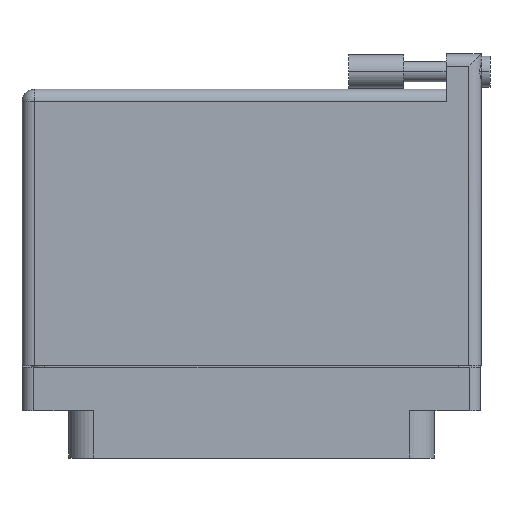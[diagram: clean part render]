
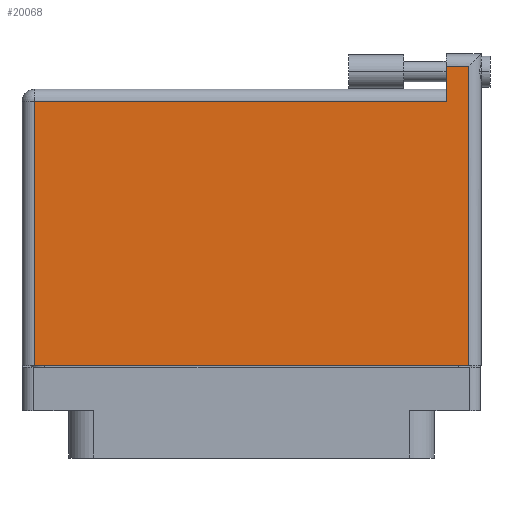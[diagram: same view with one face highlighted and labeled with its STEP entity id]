
A CAD part, front view. The second image highlights one B-rep face of the part: STEP entity #20068.
In plain terms, the highlighted face is planar.
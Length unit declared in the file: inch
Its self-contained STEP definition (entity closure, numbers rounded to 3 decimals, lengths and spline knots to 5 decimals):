
#1791 = LINE ( 'NONE', #7025, #42059 ) ;
#1835 = EDGE_CURVE ( 'NONE', #20853, #13419, #1791, .T. ) ;
#2866 = CARTESIAN_POINT ( 'NONE',  ( -1.23, -0.1, 0.4495 ) ) ;
#3007 = DIRECTION ( 'NONE',  ( -1., 0., 0. ) ) ;
#3185 = CARTESIAN_POINT ( 'NONE',  ( 1.103, 1.666, 0.4495 ) ) ;
#3357 = CARTESIAN_POINT ( 'NONE',  ( -1.3, 1.396, 0.4495 ) ) ;
#3384 = CARTESIAN_POINT ( 'NONE',  ( -1.23, -0.1, 0.4495 ) ) ;
#4077 = LINE ( 'NONE', #3185, #24847 ) ;
#4227 = EDGE_CURVE ( 'NONE', #46879, #28862, #27658, .T. ) ;
#7025 = CARTESIAN_POINT ( 'NONE',  ( 1.23, 1.666, 0.4495 ) ) ;
#8072 = AXIS2_PLACEMENT_3D ( 'NONE', #17800, #40169, #3007 ) ;
#8086 = LINE ( 'NONE', #27322, #13899 ) ;
#10813 = ORIENTED_EDGE ( 'NONE', *, *, #1835, .T. ) ;
#10863 = CARTESIAN_POINT ( 'NONE',  ( 1.103, 1.596, 0.4495 ) ) ;
#12463 = ORIENTED_EDGE ( 'NONE', *, *, #25154, .T. ) ;
#13419 = VERTEX_POINT ( 'NONE', #16685 ) ;
#13827 = VECTOR ( 'NONE', #18204, 39.37008 ) ;
#13899 = VECTOR ( 'NONE', #15803, 39.37008 ) ;
#14167 = EDGE_CURVE ( 'NONE', #28862, #20853, #8086, .T. ) ;
#14782 = DIRECTION ( 'NONE',  ( -1., 0., 0. ) ) ;
#15422 = CARTESIAN_POINT ( 'NONE',  ( 1.103, 1.396, 0.4495 ) ) ;
#15803 = DIRECTION ( 'NONE',  ( 1., 0., 0. ) ) ;
#16492 = ORIENTED_EDGE ( 'NONE', *, *, #32239, .T. ) ;
#16685 = CARTESIAN_POINT ( 'NONE',  ( 1.23, 1.596, 0.4495 ) ) ;
#17204 = VECTOR ( 'NONE', #17822, 39.37008 ) ;
#17800 = CARTESIAN_POINT ( 'NONE',  ( -1.3, 1.466, 0.4495 ) ) ;
#17822 = DIRECTION ( 'NONE',  ( 0., -1., 0. ) ) ;
#18204 = DIRECTION ( 'NONE',  ( -1., 0., 0. ) ) ;
#20068 = ADVANCED_FACE ( 'NONE', ( #42733 ), #47520, .F. ) ;
#20853 = VERTEX_POINT ( 'NONE', #40884 ) ;
#21132 = EDGE_CURVE ( 'NONE', #31483, #46879, #25778, .T. ) ;
#21756 = DIRECTION ( 'NONE',  ( 0., -1., 0. ) ) ;
#24600 = VECTOR ( 'NONE', #14782, 39.37008 ) ;
#24847 = VECTOR ( 'NONE', #21756, 39.37008 ) ;
#25154 = EDGE_CURVE ( 'NONE', #13419, #32241, #35807, .T. ) ;
#25505 = CARTESIAN_POINT ( 'NONE',  ( -1.23, 1.396, 0.4495 ) ) ;
#25778 = LINE ( 'NONE', #3357, #24600 ) ;
#27322 = CARTESIAN_POINT ( 'NONE',  ( -1.3, -0.1, 0.4495 ) ) ;
#27658 = LINE ( 'NONE', #2866, #17204 ) ;
#28503 = ORIENTED_EDGE ( 'NONE', *, *, #21132, .T. ) ;
#28862 = VERTEX_POINT ( 'NONE', #3384 ) ;
#29709 = CARTESIAN_POINT ( 'NONE',  ( -1.3, 1.596, 0.4495 ) ) ;
#31483 = VERTEX_POINT ( 'NONE', #15422 ) ;
#32239 = EDGE_CURVE ( 'NONE', #32241, #31483, #4077, .T. ) ;
#32241 = VERTEX_POINT ( 'NONE', #10863 ) ;
#35267 = EDGE_LOOP ( 'NONE', ( #39686, #10813, #12463, #16492, #28503, #40948 ) ) ;
#35807 = LINE ( 'NONE', #29709, #13827 ) ;
#39686 = ORIENTED_EDGE ( 'NONE', *, *, #14167, .T. ) ;
#40169 = DIRECTION ( 'NONE',  ( 0., 0., -1. ) ) ;
#40884 = CARTESIAN_POINT ( 'NONE',  ( 1.23, -0.1, 0.4495 ) ) ;
#40948 = ORIENTED_EDGE ( 'NONE', *, *, #4227, .T. ) ;
#42059 = VECTOR ( 'NONE', #44010, 39.37008 ) ;
#42733 = FACE_OUTER_BOUND ( 'NONE', #35267, .T. ) ;
#44010 = DIRECTION ( 'NONE',  ( 0., 1., 0. ) ) ;
#46879 = VERTEX_POINT ( 'NONE', #25505 ) ;
#47520 = PLANE ( 'NONE',  #8072 ) ;
